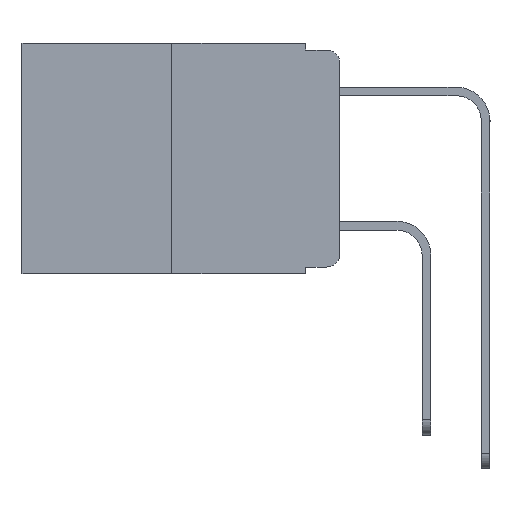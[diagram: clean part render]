
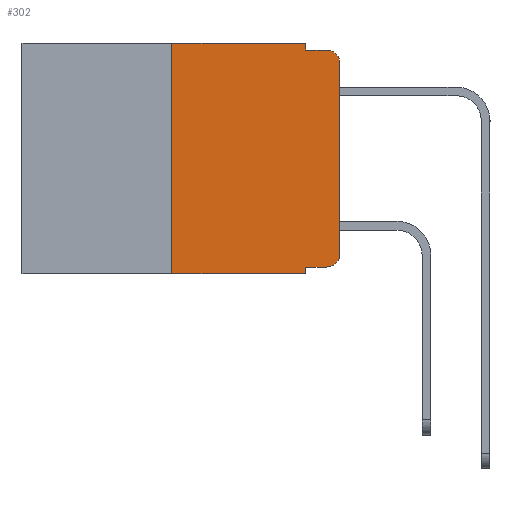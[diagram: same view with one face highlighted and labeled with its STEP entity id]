
A CAD part, left-side view. The second image highlights one B-rep face of the part: STEP entity #302.
In plain terms, the highlighted planar face has unit normal (-1, 0, 0).
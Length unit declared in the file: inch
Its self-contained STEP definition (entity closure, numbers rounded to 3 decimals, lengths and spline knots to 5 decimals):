
#134 = VERTEX_POINT ( 'NONE', #20295 ) ;
#170 = ORIENTED_EDGE ( 'NONE', *, *, #20274, .F. ) ;
#302 = ADVANCED_FACE ( 'NONE', ( #6602 ), #15704, .F. ) ;
#349 = CARTESIAN_POINT ( 'NONE',  ( 0., 0.02, -0.03 ) ) ;
#564 = VERTEX_POINT ( 'NONE', #18052 ) ;
#800 = CARTESIAN_POINT ( 'NONE',  ( 0., 0.25, 0. ) ) ;
#821 = DIRECTION ( 'NONE',  ( 0., -1., 0. ) ) ;
#861 = VERTEX_POINT ( 'NONE', #4633 ) ;
#1049 = VERTEX_POINT ( 'NONE', #5250 ) ;
#1239 = ORIENTED_EDGE ( 'NONE', *, *, #17159, .T. ) ;
#1300 = ORIENTED_EDGE ( 'NONE', *, *, #2802, .T. ) ;
#1316 = EDGE_CURVE ( 'NONE', #1049, #8761, #3533, .T. ) ;
#1343 = EDGE_LOOP ( 'NONE', ( #1239, #4810, #170, #11985, #19730, #9704, #18315, #17175, #4917, #1300 ) ) ;
#1767 = CARTESIAN_POINT ( 'NONE',  ( 0., 0.25, -0.343 ) ) ;
#2111 = DIRECTION ( 'NONE',  ( 0., 0., -1. ) ) ;
#2135 = AXIS2_PLACEMENT_3D ( 'NONE', #349, #11663, #2111 ) ;
#2802 = EDGE_CURVE ( 'NONE', #861, #564, #19813, .T. ) ;
#2828 = CARTESIAN_POINT ( 'NONE',  ( 0., 0.051, -0.333 ) ) ;
#2878 = VECTOR ( 'NONE', #6033, 39.37008 ) ;
#3483 = EDGE_CURVE ( 'NONE', #134, #5098, #12332, .T. ) ;
#3533 = LINE ( 'NONE', #14934, #19649 ) ;
#4180 = LINE ( 'NONE', #17931, #15692 ) ;
#4515 = AXIS2_PLACEMENT_3D ( 'NONE', #18517, #18287, #18086 ) ;
#4633 = CARTESIAN_POINT ( 'NONE',  ( 0., 0.02, -0.333 ) ) ;
#4810 = ORIENTED_EDGE ( 'NONE', *, *, #3483, .T. ) ;
#4917 = ORIENTED_EDGE ( 'NONE', *, *, #17396, .T. ) ;
#5098 = VERTEX_POINT ( 'NONE', #9491 ) ;
#5250 = CARTESIAN_POINT ( 'NONE',  ( 0., 0.051, 0. ) ) ;
#5718 = LINE ( 'NONE', #19732, #9851 ) ;
#6033 = DIRECTION ( 'NONE',  ( 0., -1., 0. ) ) ;
#6547 = VERTEX_POINT ( 'NONE', #19263 ) ;
#6602 = FACE_OUTER_BOUND ( 'NONE', #1343, .T. ) ;
#6767 = DIRECTION ( 'NONE',  ( 0., 0., -1. ) ) ;
#7517 = CARTESIAN_POINT ( 'NONE',  ( 0., 0.473, -0.343 ) ) ;
#7763 = VERTEX_POINT ( 'NONE', #11389 ) ;
#8240 = LINE ( 'NONE', #7517, #16523 ) ;
#8761 = VERTEX_POINT ( 'NONE', #20222 ) ;
#9002 = CARTESIAN_POINT ( 'NONE',  ( 0., 0.25, 0. ) ) ;
#9491 = CARTESIAN_POINT ( 'NONE',  ( 0., 0.02, -0.01 ) ) ;
#9704 = ORIENTED_EDGE ( 'NONE', *, *, #10542, .F. ) ;
#9851 = VECTOR ( 'NONE', #821, 39.37008 ) ;
#9933 = VECTOR ( 'NONE', #16840, 39.37008 ) ;
#10320 = DIRECTION ( 'NONE',  ( 0., -1., 0. ) ) ;
#10542 = EDGE_CURVE ( 'NONE', #11424, #17303, #17343, .T. ) ;
#11389 = CARTESIAN_POINT ( 'NONE',  ( 0., 0.051, -0.343 ) ) ;
#11424 = VERTEX_POINT ( 'NONE', #1767 ) ;
#11498 = DIRECTION ( 'NONE',  ( 1., 0., 0. ) ) ;
#11663 = DIRECTION ( 'NONE',  ( -1., 0., 0. ) ) ;
#11985 = ORIENTED_EDGE ( 'NONE', *, *, #1316, .F. ) ;
#12332 = CIRCLE ( 'NONE', #2135, 0.02 ) ;
#13096 = EDGE_CURVE ( 'NONE', #11424, #7763, #8240, .T. ) ;
#13678 = AXIS2_PLACEMENT_3D ( 'NONE', #20134, #11498, #15640 ) ;
#14934 = CARTESIAN_POINT ( 'NONE',  ( 0., 0.051, 0. ) ) ;
#15299 = CARTESIAN_POINT ( 'NONE',  ( 0., 0.051, 0. ) ) ;
#15640 = DIRECTION ( 'NONE',  ( 0., 0., -1. ) ) ;
#15692 = VECTOR ( 'NONE', #19449, 39.37008 ) ;
#15704 = PLANE ( 'NONE',  #13678 ) ;
#16046 = LINE ( 'NONE', #19569, #19624 ) ;
#16523 = VECTOR ( 'NONE', #18393, 39.37008 ) ;
#16603 = EDGE_CURVE ( 'NONE', #17303, #1049, #5718, .T. ) ;
#16840 = DIRECTION ( 'NONE',  ( 0., 0., -1. ) ) ;
#17159 = EDGE_CURVE ( 'NONE', #564, #134, #4180, .T. ) ;
#17175 = ORIENTED_EDGE ( 'NONE', *, *, #20394, .F. ) ;
#17303 = VERTEX_POINT ( 'NONE', #800 ) ;
#17343 = LINE ( 'NONE', #9002, #18317 ) ;
#17396 = EDGE_CURVE ( 'NONE', #6547, #861, #19969, .T. ) ;
#17722 = LINE ( 'NONE', #15299, #9933 ) ;
#17931 = CARTESIAN_POINT ( 'NONE',  ( 0., 0., 0. ) ) ;
#18052 = CARTESIAN_POINT ( 'NONE',  ( 0., 0., -0.313 ) ) ;
#18086 = DIRECTION ( 'NONE',  ( 0., 0., -1. ) ) ;
#18287 = DIRECTION ( 'NONE',  ( -1., 0., 0. ) ) ;
#18315 = ORIENTED_EDGE ( 'NONE', *, *, #13096, .T. ) ;
#18317 = VECTOR ( 'NONE', #19803, 39.37008 ) ;
#18393 = DIRECTION ( 'NONE',  ( 0., -1., 0. ) ) ;
#18517 = CARTESIAN_POINT ( 'NONE',  ( 0., 0.02, -0.313 ) ) ;
#19263 = CARTESIAN_POINT ( 'NONE',  ( 0., 0.051, -0.333 ) ) ;
#19449 = DIRECTION ( 'NONE',  ( 0., 0., 1. ) ) ;
#19569 = CARTESIAN_POINT ( 'NONE',  ( 0., 0.051, -0.01 ) ) ;
#19624 = VECTOR ( 'NONE', #10320, 39.37008 ) ;
#19649 = VECTOR ( 'NONE', #6767, 39.37008 ) ;
#19730 = ORIENTED_EDGE ( 'NONE', *, *, #16603, .F. ) ;
#19732 = CARTESIAN_POINT ( 'NONE',  ( 0., 0.473, 0. ) ) ;
#19803 = DIRECTION ( 'NONE',  ( 0., 0., 1. ) ) ;
#19813 = CIRCLE ( 'NONE', #4515, 0.02 ) ;
#19969 = LINE ( 'NONE', #2828, #2878 ) ;
#20134 = CARTESIAN_POINT ( 'NONE',  ( 0., 0.473, 0. ) ) ;
#20222 = CARTESIAN_POINT ( 'NONE',  ( 0., 0.051, -0.01 ) ) ;
#20274 = EDGE_CURVE ( 'NONE', #8761, #5098, #16046, .T. ) ;
#20295 = CARTESIAN_POINT ( 'NONE',  ( 0., 0., -0.03 ) ) ;
#20394 = EDGE_CURVE ( 'NONE', #6547, #7763, #17722, .T. ) ;
